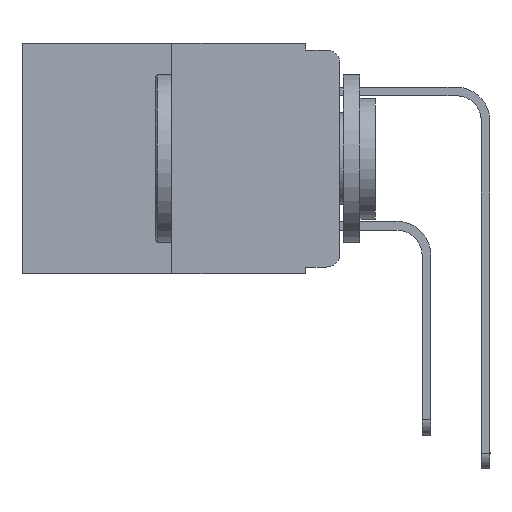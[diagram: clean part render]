
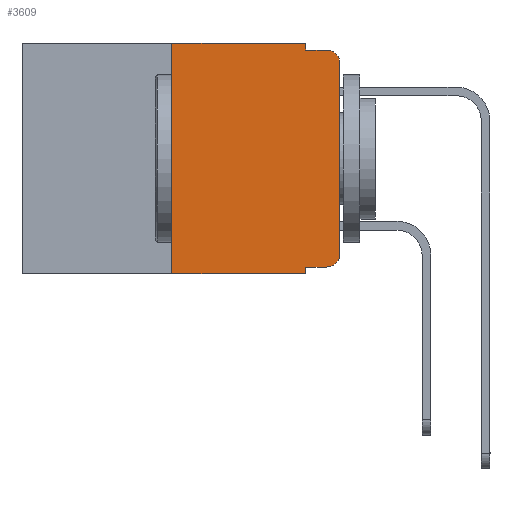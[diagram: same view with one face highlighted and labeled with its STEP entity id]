
A CAD part, left-side view. The second image highlights one B-rep face of the part: STEP entity #3609.
In plain terms, the highlighted planar face has unit normal (-1, 0, 0).
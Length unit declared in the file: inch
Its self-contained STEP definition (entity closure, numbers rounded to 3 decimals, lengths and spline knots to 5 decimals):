
#544 = DIRECTION ( 'NONE',  ( 0., 0., -1. ) ) ;
#546 = VERTEX_POINT ( 'NONE', #1733 ) ;
#619 = EDGE_CURVE ( 'NONE', #546, #2240, #6845, .T. ) ;
#651 = CARTESIAN_POINT ( 'NONE',  ( 0., 0.473, -0.343 ) ) ;
#706 = CARTESIAN_POINT ( 'NONE',  ( 0., 0.25, -0.343 ) ) ;
#753 = CARTESIAN_POINT ( 'NONE',  ( 0., 0.051, -0.333 ) ) ;
#804 = AXIS2_PLACEMENT_3D ( 'NONE', #1659, #1592, #13346 ) ;
#964 = EDGE_CURVE ( 'NONE', #2240, #1736, #1642, .T. ) ;
#973 = CARTESIAN_POINT ( 'NONE',  ( 0., 0.473, 0. ) ) ;
#1143 = ORIENTED_EDGE ( 'NONE', *, *, #8077, .F. ) ;
#1592 = DIRECTION ( 'NONE',  ( -1., 0., 0. ) ) ;
#1642 = LINE ( 'NONE', #11308, #2775 ) ;
#1659 = CARTESIAN_POINT ( 'NONE',  ( 0., 0.02, -0.313 ) ) ;
#1733 = CARTESIAN_POINT ( 'NONE',  ( 0., 0.02, -0.333 ) ) ;
#1736 = VERTEX_POINT ( 'NONE', #9658 ) ;
#1831 = CIRCLE ( 'NONE', #9214, 0.02 ) ;
#2064 = ORIENTED_EDGE ( 'NONE', *, *, #5828, .F. ) ;
#2240 = VERTEX_POINT ( 'NONE', #9574 ) ;
#2481 = DIRECTION ( 'NONE',  ( 0., 0., 1. ) ) ;
#2520 = VECTOR ( 'NONE', #9782, 39.37008 ) ;
#2763 = VERTEX_POINT ( 'NONE', #9415 ) ;
#2775 = VECTOR ( 'NONE', #3754, 39.37008 ) ;
#2797 = LINE ( 'NONE', #5952, #3416 ) ;
#3416 = VECTOR ( 'NONE', #544, 39.37008 ) ;
#3464 = CARTESIAN_POINT ( 'NONE',  ( 0., 0.25, 0. ) ) ;
#3524 = CARTESIAN_POINT ( 'NONE',  ( 0., 0.02, -0.03 ) ) ;
#3527 = VERTEX_POINT ( 'NONE', #8252 ) ;
#3609 = ADVANCED_FACE ( 'NONE', ( #7337 ), #6305, .F. ) ;
#3754 = DIRECTION ( 'NONE',  ( 0., 0., 1. ) ) ;
#4432 = LINE ( 'NONE', #6453, #6987 ) ;
#4524 = ORIENTED_EDGE ( 'NONE', *, *, #12463, .F. ) ;
#4814 = VECTOR ( 'NONE', #8092, 39.37008 ) ;
#4888 = LINE ( 'NONE', #13410, #4814 ) ;
#4933 = DIRECTION ( 'NONE',  ( 0., -1., 0. ) ) ;
#5148 = ORIENTED_EDGE ( 'NONE', *, *, #7004, .T. ) ;
#5709 = DIRECTION ( 'NONE',  ( -1., 0., 0. ) ) ;
#5828 = EDGE_CURVE ( 'NONE', #7077, #7254, #11995, .T. ) ;
#5952 = CARTESIAN_POINT ( 'NONE',  ( 0., 0.051, 0. ) ) ;
#6093 = VECTOR ( 'NONE', #4933, 39.37008 ) ;
#6150 = ORIENTED_EDGE ( 'NONE', *, *, #619, .T. ) ;
#6189 = LINE ( 'NONE', #651, #6093 ) ;
#6305 = PLANE ( 'NONE',  #9726 ) ;
#6453 = CARTESIAN_POINT ( 'NONE',  ( 0., 0.051, -0.333 ) ) ;
#6845 = CIRCLE ( 'NONE', #804, 0.02 ) ;
#6987 = VECTOR ( 'NONE', #10721, 39.37008 ) ;
#7004 = EDGE_CURVE ( 'NONE', #1736, #3527, #1831, .T. ) ;
#7077 = VERTEX_POINT ( 'NONE', #11422 ) ;
#7170 = ORIENTED_EDGE ( 'NONE', *, *, #964, .T. ) ;
#7178 = EDGE_CURVE ( 'NONE', #9007, #2763, #6189, .T. ) ;
#7254 = VERTEX_POINT ( 'NONE', #7557 ) ;
#7337 = FACE_OUTER_BOUND ( 'NONE', #8250, .T. ) ;
#7381 = VECTOR ( 'NONE', #8568, 39.37008 ) ;
#7418 = EDGE_CURVE ( 'NONE', #8038, #546, #4432, .T. ) ;
#7541 = DIRECTION ( 'NONE',  ( 1., 0., 0. ) ) ;
#7557 = CARTESIAN_POINT ( 'NONE',  ( 0., 0.051, -0.01 ) ) ;
#7897 = LINE ( 'NONE', #8795, #2520 ) ;
#7947 = EDGE_CURVE ( 'NONE', #10872, #7077, #7897, .T. ) ;
#8031 = ORIENTED_EDGE ( 'NONE', *, *, #7947, .F. ) ;
#8038 = VERTEX_POINT ( 'NONE', #753 ) ;
#8077 = EDGE_CURVE ( 'NONE', #8038, #2763, #2797, .T. ) ;
#8092 = DIRECTION ( 'NONE',  ( 0., -1., 0. ) ) ;
#8250 = EDGE_LOOP ( 'NONE', ( #7170, #5148, #9467, #2064, #8031, #4524, #8509, #1143, #8342, #6150 ) ) ;
#8252 = CARTESIAN_POINT ( 'NONE',  ( 0., 0.02, -0.01 ) ) ;
#8342 = ORIENTED_EDGE ( 'NONE', *, *, #7418, .T. ) ;
#8509 = ORIENTED_EDGE ( 'NONE', *, *, #7178, .T. ) ;
#8568 = DIRECTION ( 'NONE',  ( 0., 0., -1. ) ) ;
#8795 = CARTESIAN_POINT ( 'NONE',  ( 0., 0.473, 0. ) ) ;
#9007 = VERTEX_POINT ( 'NONE', #706 ) ;
#9214 = AXIS2_PLACEMENT_3D ( 'NONE', #3524, #5709, #9963 ) ;
#9287 = CARTESIAN_POINT ( 'NONE',  ( 0., 0.25, 0. ) ) ;
#9415 = CARTESIAN_POINT ( 'NONE',  ( 0., 0.051, -0.343 ) ) ;
#9467 = ORIENTED_EDGE ( 'NONE', *, *, #9775, .F. ) ;
#9518 = DIRECTION ( 'NONE',  ( 0., 0., -1. ) ) ;
#9574 = CARTESIAN_POINT ( 'NONE',  ( 0., 0., -0.313 ) ) ;
#9618 = CARTESIAN_POINT ( 'NONE',  ( 0., 0.051, 0. ) ) ;
#9658 = CARTESIAN_POINT ( 'NONE',  ( 0., 0., -0.03 ) ) ;
#9726 = AXIS2_PLACEMENT_3D ( 'NONE', #973, #7541, #9518 ) ;
#9775 = EDGE_CURVE ( 'NONE', #7254, #3527, #4888, .T. ) ;
#9782 = DIRECTION ( 'NONE',  ( 0., -1., 0. ) ) ;
#9963 = DIRECTION ( 'NONE',  ( 0., 0., -1. ) ) ;
#10046 = LINE ( 'NONE', #3464, #11323 ) ;
#10721 = DIRECTION ( 'NONE',  ( 0., -1., 0. ) ) ;
#10872 = VERTEX_POINT ( 'NONE', #9287 ) ;
#11308 = CARTESIAN_POINT ( 'NONE',  ( 0., 0., 0. ) ) ;
#11323 = VECTOR ( 'NONE', #2481, 39.37008 ) ;
#11422 = CARTESIAN_POINT ( 'NONE',  ( 0., 0.051, 0. ) ) ;
#11995 = LINE ( 'NONE', #9618, #7381 ) ;
#12463 = EDGE_CURVE ( 'NONE', #9007, #10872, #10046, .T. ) ;
#13346 = DIRECTION ( 'NONE',  ( 0., 0., -1. ) ) ;
#13410 = CARTESIAN_POINT ( 'NONE',  ( 0., 0.051, -0.01 ) ) ;
